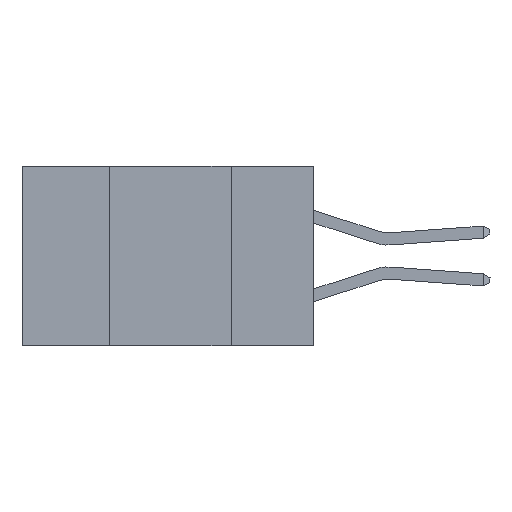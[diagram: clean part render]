
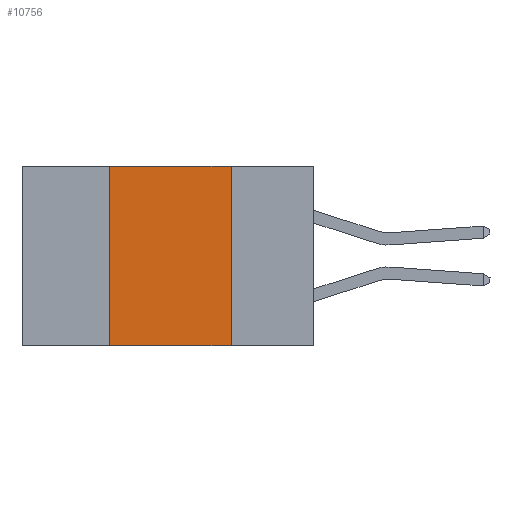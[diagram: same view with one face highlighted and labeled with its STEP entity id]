
A CAD part, left-side view. The second image highlights one B-rep face of the part: STEP entity #10756.
In plain terms, the highlighted planar face has unit normal (-1, 0, 0).
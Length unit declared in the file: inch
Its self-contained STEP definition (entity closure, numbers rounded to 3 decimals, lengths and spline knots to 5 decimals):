
#115 = CARTESIAN_POINT ( 'NONE',  ( 0., 0.42, -0.37 ) ) ;
#205 = DIRECTION ( 'NONE',  ( 0., -1., 0. ) ) ;
#374 = CARTESIAN_POINT ( 'NONE',  ( 0., 0.6, 0. ) ) ;
#1208 = ORIENTED_EDGE ( 'NONE', *, *, #8018, .F. ) ;
#1421 = DIRECTION ( 'NONE',  ( 0., 0., 1. ) ) ;
#1515 = DIRECTION ( 'NONE',  ( 1., 0., 0. ) ) ;
#1586 = AXIS2_PLACEMENT_3D ( 'NONE', #374, #1515, #8841 ) ;
#1597 = VECTOR ( 'NONE', #205, 39.37008 ) ;
#2221 = ORIENTED_EDGE ( 'NONE', *, *, #6257, .T. ) ;
#2276 = VECTOR ( 'NONE', #10547, 39.37008 ) ;
#2404 = LINE ( 'NONE', #2447, #13124 ) ;
#2447 = CARTESIAN_POINT ( 'NONE',  ( 0., 0.42, 0. ) ) ;
#3057 = DIRECTION ( 'NONE',  ( 0., -1., 0. ) ) ;
#3182 = CARTESIAN_POINT ( 'NONE',  ( 0., 0.17, 0. ) ) ;
#3183 = EDGE_CURVE ( 'NONE', #8047, #6754, #5721, .T. ) ;
#3351 = VERTEX_POINT ( 'NONE', #115 ) ;
#3623 = CARTESIAN_POINT ( 'NONE',  ( 0., 0.17, -0.37 ) ) ;
#4241 = CARTESIAN_POINT ( 'NONE',  ( 0., 0.17, 0. ) ) ;
#4481 = CARTESIAN_POINT ( 'NONE',  ( 0., 0.6, -0.37 ) ) ;
#5721 = LINE ( 'NONE', #13403, #11341 ) ;
#6257 = EDGE_CURVE ( 'NONE', #3351, #10761, #12691, .T. ) ;
#6670 = EDGE_LOOP ( 'NONE', ( #1208, #12345, #7120, #2221 ) ) ;
#6741 = PLANE ( 'NONE',  #1586 ) ;
#6754 = VERTEX_POINT ( 'NONE', #4241 ) ;
#6893 = EDGE_CURVE ( 'NONE', #3351, #8047, #2404, .T. ) ;
#7120 = ORIENTED_EDGE ( 'NONE', *, *, #6893, .F. ) ;
#7499 = LINE ( 'NONE', #3182, #2276 ) ;
#8018 = EDGE_CURVE ( 'NONE', #6754, #10761, #7499, .T. ) ;
#8047 = VERTEX_POINT ( 'NONE', #8635 ) ;
#8635 = CARTESIAN_POINT ( 'NONE',  ( 0., 0.42, 0. ) ) ;
#8841 = DIRECTION ( 'NONE',  ( 0., 0., -1. ) ) ;
#8931 = FACE_OUTER_BOUND ( 'NONE', #6670, .T. ) ;
#10547 = DIRECTION ( 'NONE',  ( 0., 0., -1. ) ) ;
#10756 = ADVANCED_FACE ( 'NONE', ( #8931 ), #6741, .F. ) ;
#10761 = VERTEX_POINT ( 'NONE', #3623 ) ;
#11341 = VECTOR ( 'NONE', #3057, 39.37008 ) ;
#12345 = ORIENTED_EDGE ( 'NONE', *, *, #3183, .F. ) ;
#12691 = LINE ( 'NONE', #4481, #1597 ) ;
#13124 = VECTOR ( 'NONE', #1421, 39.37008 ) ;
#13403 = CARTESIAN_POINT ( 'NONE',  ( 0., 0.6, 0. ) ) ;
